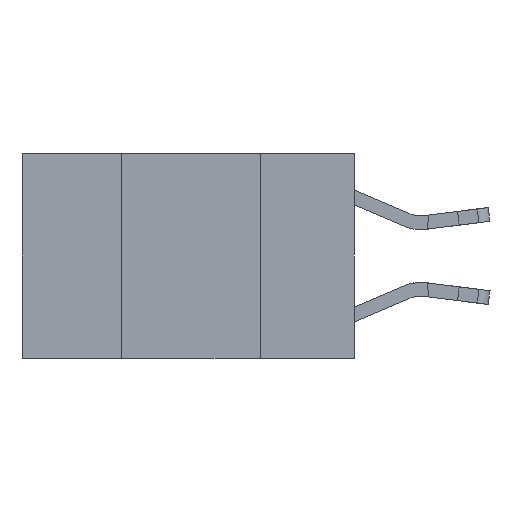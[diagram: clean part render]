
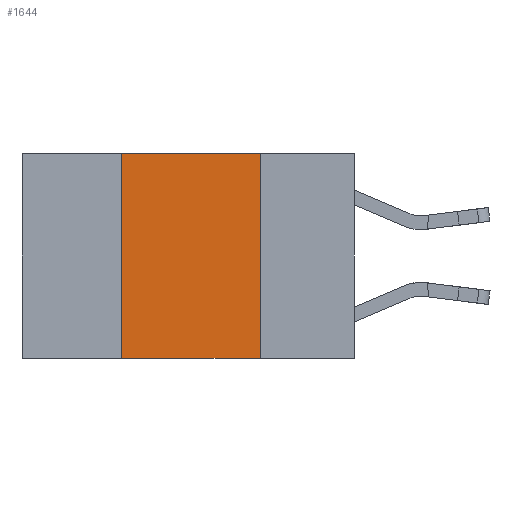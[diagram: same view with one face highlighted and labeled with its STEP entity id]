
A CAD part, left-side view. The second image highlights one B-rep face of the part: STEP entity #1644.
In plain terms, the highlighted planar face has unit normal (-1, 0, 0).
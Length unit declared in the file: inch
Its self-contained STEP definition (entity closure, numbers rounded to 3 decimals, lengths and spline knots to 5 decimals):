
#434 = EDGE_CURVE ( 'NONE', #2634, #25431, #10058, .T. ) ;
#1644 = ADVANCED_FACE ( 'NONE', ( #27975 ), #12969, .F. ) ;
#1878 = VECTOR ( 'NONE', #12266, 39.37008 ) ;
#2055 = DIRECTION ( 'NONE',  ( 0., -1., 0. ) ) ;
#2519 = EDGE_LOOP ( 'NONE', ( #21703, #10456, #11875, #6564 ) ) ;
#2571 = LINE ( 'NONE', #18961, #1878 ) ;
#2634 = VERTEX_POINT ( 'NONE', #4823 ) ;
#3709 = CARTESIAN_POINT ( 'NONE',  ( 0., 0.42, -0.37 ) ) ;
#3931 = DIRECTION ( 'NONE',  ( 0., 0., -1. ) ) ;
#4823 = CARTESIAN_POINT ( 'NONE',  ( 0., 0.42, 0. ) ) ;
#5700 = CARTESIAN_POINT ( 'NONE',  ( 0., 0.42, 0. ) ) ;
#6403 = EDGE_CURVE ( 'NONE', #10332, #2634, #7036, .T. ) ;
#6564 = ORIENTED_EDGE ( 'NONE', *, *, #10571, .T. ) ;
#7036 = LINE ( 'NONE', #5700, #18344 ) ;
#7592 = CARTESIAN_POINT ( 'NONE',  ( 0., 0.17, 0. ) ) ;
#7994 = DIRECTION ( 'NONE',  ( 0., 0., 1. ) ) ;
#9160 = CARTESIAN_POINT ( 'NONE',  ( 0., 0.6, -0.37 ) ) ;
#9881 = CARTESIAN_POINT ( 'NONE',  ( 0., 0.17, -0.37 ) ) ;
#10058 = LINE ( 'NONE', #17874, #22019 ) ;
#10332 = VERTEX_POINT ( 'NONE', #3709 ) ;
#10456 = ORIENTED_EDGE ( 'NONE', *, *, #434, .F. ) ;
#10571 = EDGE_CURVE ( 'NONE', #10332, #12031, #11800, .T. ) ;
#11800 = LINE ( 'NONE', #9160, #17096 ) ;
#11875 = ORIENTED_EDGE ( 'NONE', *, *, #6403, .F. ) ;
#12031 = VERTEX_POINT ( 'NONE', #9881 ) ;
#12266 = DIRECTION ( 'NONE',  ( 0., 0., -1. ) ) ;
#12969 = PLANE ( 'NONE',  #21249 ) ;
#15229 = CARTESIAN_POINT ( 'NONE',  ( 0., 0.6, 0. ) ) ;
#17096 = VECTOR ( 'NONE', #27086, 39.37008 ) ;
#17520 = DIRECTION ( 'NONE',  ( 1., 0., 0. ) ) ;
#17874 = CARTESIAN_POINT ( 'NONE',  ( 0., 0.6, 0. ) ) ;
#18344 = VECTOR ( 'NONE', #7994, 39.37008 ) ;
#18961 = CARTESIAN_POINT ( 'NONE',  ( 0., 0.17, 0. ) ) ;
#19071 = EDGE_CURVE ( 'NONE', #25431, #12031, #2571, .T. ) ;
#21249 = AXIS2_PLACEMENT_3D ( 'NONE', #15229, #17520, #3931 ) ;
#21703 = ORIENTED_EDGE ( 'NONE', *, *, #19071, .F. ) ;
#22019 = VECTOR ( 'NONE', #2055, 39.37008 ) ;
#25431 = VERTEX_POINT ( 'NONE', #7592 ) ;
#27086 = DIRECTION ( 'NONE',  ( 0., -1., 0. ) ) ;
#27975 = FACE_OUTER_BOUND ( 'NONE', #2519, .T. ) ;
